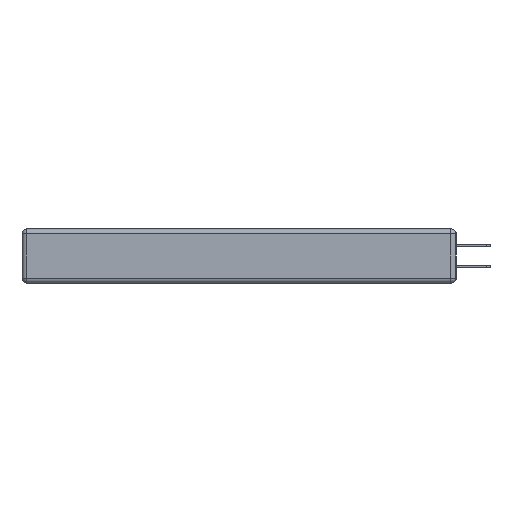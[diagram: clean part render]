
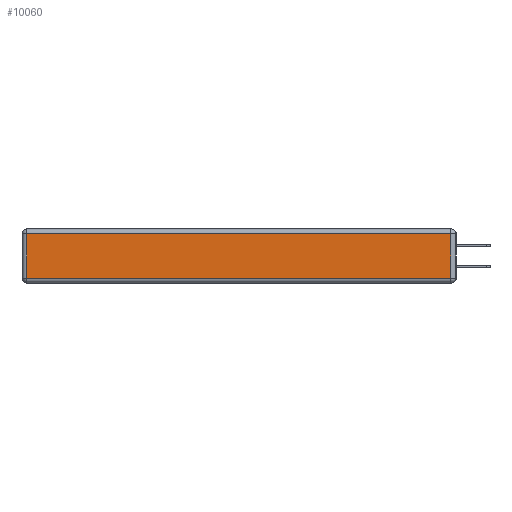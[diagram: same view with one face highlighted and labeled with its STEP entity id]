
A CAD part, left-side view. The second image highlights one B-rep face of the part: STEP entity #10060.
In plain terms, the highlighted planar face has unit normal (-1, 0, 0).
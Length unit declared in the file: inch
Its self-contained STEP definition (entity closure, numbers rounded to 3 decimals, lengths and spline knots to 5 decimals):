
#179 = CARTESIAN_POINT ( 'NONE',  ( 0., 2.75, -0.03 ) ) ;
#417 = DIRECTION ( 'NONE',  ( 0., -1., 0. ) ) ;
#893 = CARTESIAN_POINT ( 'NONE',  ( 0., 0., -0.313 ) ) ;
#1313 = ORIENTED_EDGE ( 'NONE', *, *, #15729, .T. ) ;
#2184 = LINE ( 'NONE', #6781, #10613 ) ;
#2308 = ORIENTED_EDGE ( 'NONE', *, *, #8143, .T. ) ;
#3061 = CARTESIAN_POINT ( 'NONE',  ( 0., 0., -0.343 ) ) ;
#3148 = CARTESIAN_POINT ( 'NONE',  ( 0., 0.03, -0.03 ) ) ;
#3884 = FACE_OUTER_BOUND ( 'NONE', #13178, .T. ) ;
#4079 = CARTESIAN_POINT ( 'NONE',  ( 0., 2.72, -0.03 ) ) ;
#4231 = ORIENTED_EDGE ( 'NONE', *, *, #13396, .T. ) ;
#5499 = CARTESIAN_POINT ( 'NONE',  ( 0., 0.03, -0.343 ) ) ;
#6766 = ORIENTED_EDGE ( 'NONE', *, *, #9348, .T. ) ;
#6781 = CARTESIAN_POINT ( 'NONE',  ( 0., 2.72, -0.343 ) ) ;
#7770 = CARTESIAN_POINT ( 'NONE',  ( 0., 0.03, -0.313 ) ) ;
#8143 = EDGE_CURVE ( 'NONE', #13335, #8743, #14162, .T. ) ;
#8344 = VECTOR ( 'NONE', #8527, 39.37008 ) ;
#8527 = DIRECTION ( 'NONE',  ( 0., 0., 1. ) ) ;
#8743 = VERTEX_POINT ( 'NONE', #4079 ) ;
#8803 = LINE ( 'NONE', #5499, #8344 ) ;
#9180 = VERTEX_POINT ( 'NONE', #12232 ) ;
#9348 = EDGE_CURVE ( 'NONE', #9640, #13335, #8803, .T. ) ;
#9640 = VERTEX_POINT ( 'NONE', #7770 ) ;
#9933 = AXIS2_PLACEMENT_3D ( 'NONE', #3061, #11560, #15874 ) ;
#10060 = ADVANCED_FACE ( 'NONE', ( #3884 ), #11615, .T. ) ;
#10148 = DIRECTION ( 'NONE',  ( 0., 1., 0. ) ) ;
#10613 = VECTOR ( 'NONE', #18062, 39.37008 ) ;
#10986 = LINE ( 'NONE', #893, #12091 ) ;
#11560 = DIRECTION ( 'NONE',  ( -1., 0., 0. ) ) ;
#11615 = PLANE ( 'NONE',  #9933 ) ;
#12091 = VECTOR ( 'NONE', #417, 39.37008 ) ;
#12232 = CARTESIAN_POINT ( 'NONE',  ( 0., 2.72, -0.313 ) ) ;
#13178 = EDGE_LOOP ( 'NONE', ( #1313, #6766, #2308, #4231 ) ) ;
#13335 = VERTEX_POINT ( 'NONE', #3148 ) ;
#13396 = EDGE_CURVE ( 'NONE', #8743, #9180, #2184, .T. ) ;
#13707 = VECTOR ( 'NONE', #10148, 39.37008 ) ;
#14162 = LINE ( 'NONE', #179, #13707 ) ;
#15729 = EDGE_CURVE ( 'NONE', #9180, #9640, #10986, .T. ) ;
#15874 = DIRECTION ( 'NONE',  ( 0., 0., 1. ) ) ;
#18062 = DIRECTION ( 'NONE',  ( 0., 0., -1. ) ) ;
